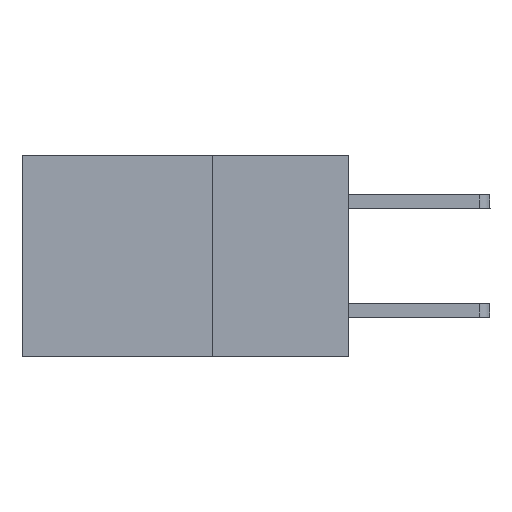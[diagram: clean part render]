
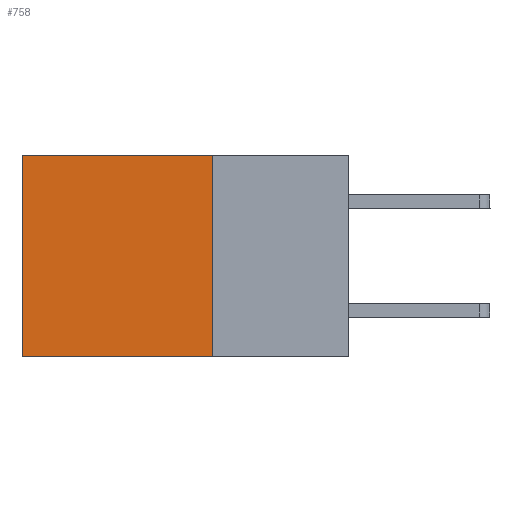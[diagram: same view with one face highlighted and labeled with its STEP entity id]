
A CAD part, left-side view. The second image highlights one B-rep face of the part: STEP entity #758.
In plain terms, the highlighted planar face has unit normal (-1, 0, 0).
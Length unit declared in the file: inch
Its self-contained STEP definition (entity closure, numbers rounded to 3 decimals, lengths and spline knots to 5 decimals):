
#76 = CARTESIAN_POINT ( 'NONE',  ( 0.298, 0.25, 0. ) ) ;
#145 = EDGE_CURVE ( 'NONE', #4986, #7769, #4182, .T. ) ;
#337 = ORIENTED_EDGE ( 'NONE', *, *, #2517, .T. ) ;
#461 = VECTOR ( 'NONE', #8590, 39.37008 ) ;
#630 = EDGE_CURVE ( 'NONE', #6633, #7769, #3285, .T. ) ;
#758 = ADVANCED_FACE ( 'NONE', ( #8989 ), #6941, .F. ) ;
#966 = CARTESIAN_POINT ( 'NONE',  ( 0.298, 0.6, -0.37 ) ) ;
#1267 = CARTESIAN_POINT ( 'NONE',  ( 0.298, 0.25, 0. ) ) ;
#1320 = VECTOR ( 'NONE', #4805, 39.37008 ) ;
#1356 = EDGE_LOOP ( 'NONE', ( #4851, #4835, #3519, #337 ) ) ;
#2091 = CARTESIAN_POINT ( 'NONE',  ( 0.298, 0.6, 0. ) ) ;
#2517 = EDGE_CURVE ( 'NONE', #4279, #4986, #8160, .T. ) ;
#2711 = CARTESIAN_POINT ( 'NONE',  ( 0.298, 0.6, 0. ) ) ;
#3285 = LINE ( 'NONE', #6134, #5189 ) ;
#3386 = CARTESIAN_POINT ( 'NONE',  ( 0.298, 0.25, 0. ) ) ;
#3512 = EDGE_CURVE ( 'NONE', #4279, #6633, #8614, .T. ) ;
#3519 = ORIENTED_EDGE ( 'NONE', *, *, #3512, .F. ) ;
#4182 = LINE ( 'NONE', #2711, #1320 ) ;
#4279 = VERTEX_POINT ( 'NONE', #6983 ) ;
#4805 = DIRECTION ( 'NONE',  ( 0., 0., -1. ) ) ;
#4835 = ORIENTED_EDGE ( 'NONE', *, *, #630, .F. ) ;
#4851 = ORIENTED_EDGE ( 'NONE', *, *, #145, .T. ) ;
#4880 = DIRECTION ( 'NONE',  ( 0., 0., -1. ) ) ;
#4986 = VERTEX_POINT ( 'NONE', #2091 ) ;
#5189 = VECTOR ( 'NONE', #6848, 39.37008 ) ;
#6134 = CARTESIAN_POINT ( 'NONE',  ( 0.298, 0.25, -0.37 ) ) ;
#6633 = VERTEX_POINT ( 'NONE', #8253 ) ;
#6695 = VECTOR ( 'NONE', #4880, 39.37008 ) ;
#6848 = DIRECTION ( 'NONE',  ( 0., 1., 0. ) ) ;
#6909 = DIRECTION ( 'NONE',  ( 1., 0., 0. ) ) ;
#6941 = PLANE ( 'NONE',  #7738 ) ;
#6983 = CARTESIAN_POINT ( 'NONE',  ( 0.298, 0.25, 0. ) ) ;
#7631 = DIRECTION ( 'NONE',  ( 0., 0., -1. ) ) ;
#7738 = AXIS2_PLACEMENT_3D ( 'NONE', #1267, #6909, #7631 ) ;
#7769 = VERTEX_POINT ( 'NONE', #966 ) ;
#8160 = LINE ( 'NONE', #76, #461 ) ;
#8253 = CARTESIAN_POINT ( 'NONE',  ( 0.298, 0.25, -0.37 ) ) ;
#8590 = DIRECTION ( 'NONE',  ( 0., 1., 0. ) ) ;
#8614 = LINE ( 'NONE', #3386, #6695 ) ;
#8989 = FACE_OUTER_BOUND ( 'NONE', #1356, .T. ) ;
